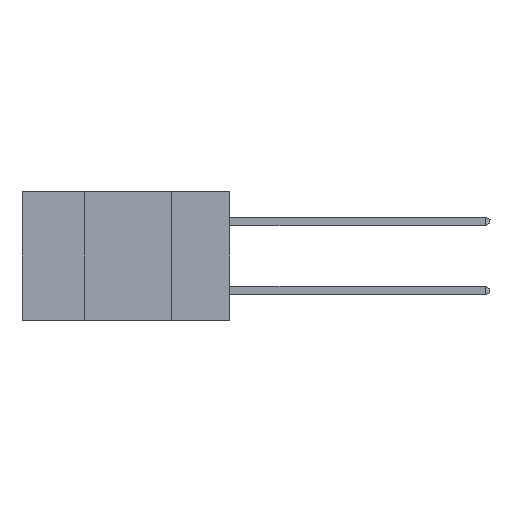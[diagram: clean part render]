
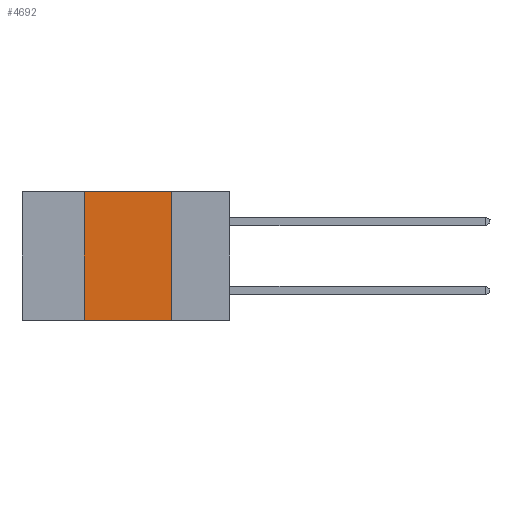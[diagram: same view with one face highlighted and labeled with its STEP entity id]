
A CAD part, left-side view. The second image highlights one B-rep face of the part: STEP entity #4692.
In plain terms, the highlighted planar face has unit normal (-1, 0, 0).
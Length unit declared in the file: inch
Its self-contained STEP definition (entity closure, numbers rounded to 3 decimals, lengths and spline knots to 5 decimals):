
#923 = DIRECTION ( 'NONE',  ( 0., 0., -1. ) ) ;
#1075 = LINE ( 'NONE', #12818, #5906 ) ;
#2330 = LINE ( 'NONE', #10811, #9056 ) ;
#2402 = ORIENTED_EDGE ( 'NONE', *, *, #17577, .F. ) ;
#3143 = VERTEX_POINT ( 'NONE', #10996 ) ;
#4123 = DIRECTION ( 'NONE',  ( 0., 0., 1. ) ) ;
#4665 = VERTEX_POINT ( 'NONE', #6889 ) ;
#4692 = ADVANCED_FACE ( 'NONE', ( #6980 ), #5220, .F. ) ;
#5220 = PLANE ( 'NONE',  #17217 ) ;
#5232 = VECTOR ( 'NONE', #16629, 39.37008 ) ;
#5906 = VECTOR ( 'NONE', #14037, 39.37008 ) ;
#6889 = CARTESIAN_POINT ( 'NONE',  ( 0., 0.17, 0. ) ) ;
#6980 = FACE_OUTER_BOUND ( 'NONE', #7006, .T. ) ;
#7006 = EDGE_LOOP ( 'NONE', ( #7763, #17882, #2402, #18095 ) ) ;
#7763 = ORIENTED_EDGE ( 'NONE', *, *, #7918, .F. ) ;
#7918 = EDGE_CURVE ( 'NONE', #4665, #15101, #2330, .T. ) ;
#8500 = LINE ( 'NONE', #15485, #8877 ) ;
#8877 = VECTOR ( 'NONE', #4123, 39.37008 ) ;
#9056 = VECTOR ( 'NONE', #9679, 39.37008 ) ;
#9219 = EDGE_CURVE ( 'NONE', #11231, #4665, #12248, .T. ) ;
#9679 = DIRECTION ( 'NONE',  ( 0., 0., -1. ) ) ;
#9992 = CARTESIAN_POINT ( 'NONE',  ( 0., 0.42, 0. ) ) ;
#10526 = EDGE_CURVE ( 'NONE', #3143, #15101, #1075, .T. ) ;
#10811 = CARTESIAN_POINT ( 'NONE',  ( 0., 0.17, -0.37 ) ) ;
#10996 = CARTESIAN_POINT ( 'NONE',  ( 0., 0.42, -0.37 ) ) ;
#11231 = VERTEX_POINT ( 'NONE', #9992 ) ;
#12248 = LINE ( 'NONE', #15408, #5232 ) ;
#12671 = DIRECTION ( 'NONE',  ( 1., 0., 0. ) ) ;
#12818 = CARTESIAN_POINT ( 'NONE',  ( 0., 0.6, -0.37 ) ) ;
#14037 = DIRECTION ( 'NONE',  ( 0., -1., 0. ) ) ;
#15101 = VERTEX_POINT ( 'NONE', #17046 ) ;
#15282 = CARTESIAN_POINT ( 'NONE',  ( 0., 0.6, 0. ) ) ;
#15408 = CARTESIAN_POINT ( 'NONE',  ( 0., 0.6, 0. ) ) ;
#15485 = CARTESIAN_POINT ( 'NONE',  ( 0., 0.42, -0.37 ) ) ;
#16629 = DIRECTION ( 'NONE',  ( 0., -1., 0. ) ) ;
#17046 = CARTESIAN_POINT ( 'NONE',  ( 0., 0.17, -0.37 ) ) ;
#17217 = AXIS2_PLACEMENT_3D ( 'NONE', #15282, #12671, #923 ) ;
#17577 = EDGE_CURVE ( 'NONE', #3143, #11231, #8500, .T. ) ;
#17882 = ORIENTED_EDGE ( 'NONE', *, *, #9219, .F. ) ;
#18095 = ORIENTED_EDGE ( 'NONE', *, *, #10526, .T. ) ;
